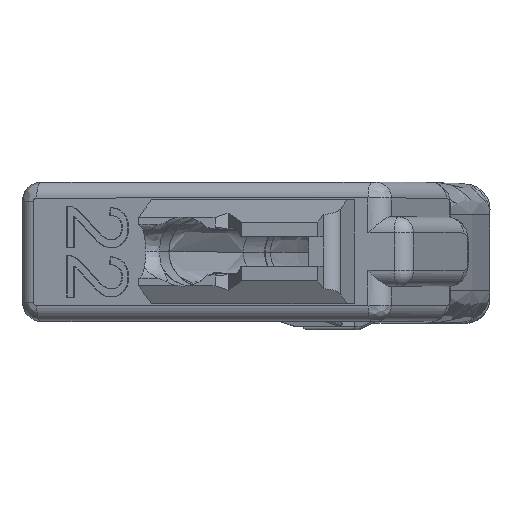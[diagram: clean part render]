
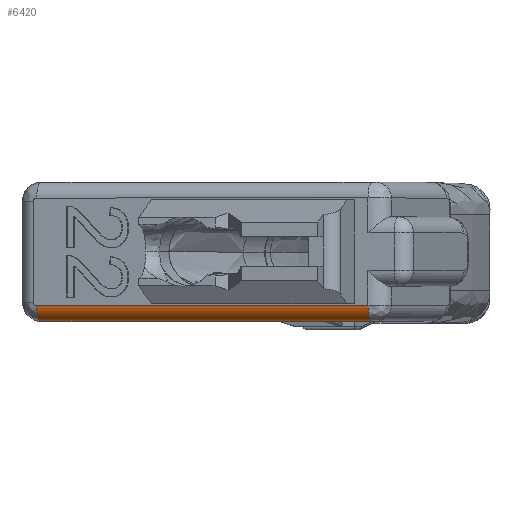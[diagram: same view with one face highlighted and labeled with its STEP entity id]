
A CAD part, top view. The second image highlights one B-rep face of the part: STEP entity #6420.
In plain terms, the highlighted cylindrical face has radius 2.5 mm (diameter 5 mm), a partial arc.
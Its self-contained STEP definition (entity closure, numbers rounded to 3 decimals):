
#101=CYLINDRICAL_SURFACE('',#6865,2.5);
#296=LINE('',#8959,#659);
#299=LINE('',#8971,#662);
#609=LINE('',#17404,#972);
#659=VECTOR('',#7002,10.);
#662=VECTOR('',#7011,10.);
#972=VECTOR('',#8033,2.5);
#1326=FACE_OUTER_BOUND('',#1700,.T.);
#1700=EDGE_LOOP('',(#5645,#5646,#5647,#5648,#5649,#5650));
#1900=CIRCLE('',#6790,2.5);
#1933=CIRCLE('',#6866,2.5);
#2312=B_SPLINE_CURVE_WITH_KNOTS('',3,(#17361,#17362,#17363,#17364,#17365,
#17366,#17367,#17368,#17369,#17370),.UNSPECIFIED.,.F.,.F.,(4,2,2,2,4),(-0.003,
0.,0.088,0.176,0.179),.UNSPECIFIED.);
#2384=VERTEX_POINT('',#8956);
#2385=VERTEX_POINT('',#8958);
#2390=VERTEX_POINT('',#8968);
#2391=VERTEX_POINT('',#8970);
#2865=VERTEX_POINT('',#15825);
#2930=VERTEX_POINT('',#17402);
#3018=EDGE_CURVE('',#2384,#2385,#296,.T.);
#3024=EDGE_CURVE('',#2391,#2390,#299,.T.);
#3742=EDGE_CURVE('',#2391,#2865,#1900,.T.);
#3876=EDGE_CURVE('',#2385,#2390,#2312,.T.);
#3888=EDGE_CURVE('',#2930,#2384,#1933,.T.);
#3889=EDGE_CURVE('',#2865,#2930,#609,.T.);
#5645=ORIENTED_EDGE('',*,*,#3888,.F.);
#5646=ORIENTED_EDGE('',*,*,#3889,.F.);
#5647=ORIENTED_EDGE('',*,*,#3742,.F.);
#5648=ORIENTED_EDGE('',*,*,#3024,.T.);
#5649=ORIENTED_EDGE('',*,*,#3876,.F.);
#5650=ORIENTED_EDGE('',*,*,#3018,.F.);
#6420=ADVANCED_FACE('',(#1326),#101,.T.);
#6790=AXIS2_PLACEMENT_3D('',#15826,#7832,#7833);
#6865=AXIS2_PLACEMENT_3D('',#17401,#8029,#8030);
#6866=AXIS2_PLACEMENT_3D('',#17403,#8031,#8032);
#7002=DIRECTION('',(-0.963,-0.106,0.247));
#7011=DIRECTION('',(0.963,0.106,-0.247));
#7832=DIRECTION('center_axis',(-0.963,-0.106,0.247));
#7833=DIRECTION('ref_axis',(0.087,-0.992,-0.087));
#8029=DIRECTION('center_axis',(0.963,0.106,-0.247));
#8030=DIRECTION('ref_axis',(0.242,-0.746,0.621));
#8031=DIRECTION('center_axis',(0.963,0.106,-0.247));
#8032=DIRECTION('ref_axis',(0.254,-0.062,0.965));
#8033=DIRECTION('',(0.963,0.106,-0.247));
#8956=CARTESIAN_POINT('',(353.92,-108.644,594.255));
#8958=CARTESIAN_POINT('',(312.662,-113.194,604.838));
#8959=CARTESIAN_POINT('',(353.716,-108.667,594.307));
#8968=CARTESIAN_POINT('',(310.903,-113.387,605.289));
#8970=CARTESIAN_POINT('',(301.705,-114.402,607.649));
#8971=CARTESIAN_POINT('',(334.148,-110.824,599.327));
#15825=CARTESIAN_POINT('',(302.123,-112.076,610.278));
#15826=CARTESIAN_POINT('Origin',(301.487,-111.921,607.866));
#17361=CARTESIAN_POINT('Ctrl Pts',(312.662,-113.194,604.838));
#17362=CARTESIAN_POINT('Ctrl Pts',(312.651,-113.195,604.842));
#17363=CARTESIAN_POINT('Ctrl Pts',(312.64,-113.196,604.845));
#17364=CARTESIAN_POINT('Ctrl Pts',(312.354,-113.23,604.943));
#17365=CARTESIAN_POINT('Ctrl Pts',(312.074,-113.261,605.027));
#17366=CARTESIAN_POINT('Ctrl Pts',(311.509,-113.324,605.172));
#17367=CARTESIAN_POINT('Ctrl Pts',(311.224,-113.354,605.233));
#17368=CARTESIAN_POINT('Ctrl Pts',(310.925,-113.385,605.285));
#17369=CARTESIAN_POINT('Ctrl Pts',(310.914,-113.386,605.287));
#17370=CARTESIAN_POINT('Ctrl Pts',(310.903,-113.387,605.289));
#17401=CARTESIAN_POINT('Origin',(333.93,-108.343,599.544));
#17402=CARTESIAN_POINT('',(354.338,-106.318,596.885));
#17403=CARTESIAN_POINT('Origin',(353.702,-106.163,594.472));
#17404=CARTESIAN_POINT('',(334.566,-108.499,601.956));
